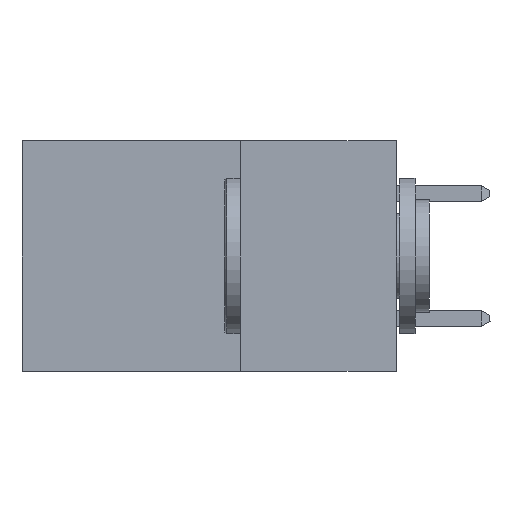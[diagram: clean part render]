
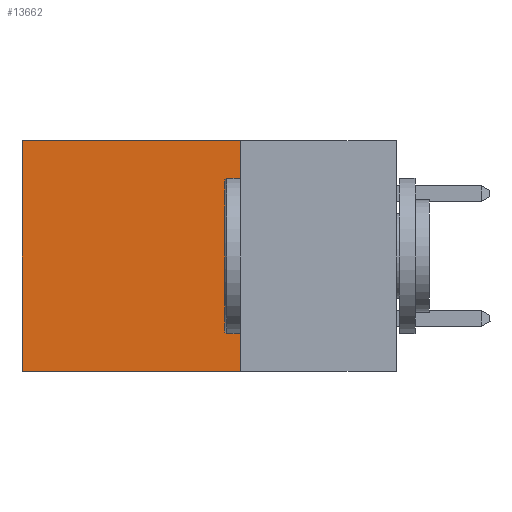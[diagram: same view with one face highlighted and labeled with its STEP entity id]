
A CAD part, left-side view. The second image highlights one B-rep face of the part: STEP entity #13662.
In plain terms, the highlighted planar face has unit normal (-1, 0, 0).
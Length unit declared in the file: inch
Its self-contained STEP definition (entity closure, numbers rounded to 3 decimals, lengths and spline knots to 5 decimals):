
#548 = LINE ( 'NONE', #16639, #19822 ) ;
#828 = PLANE ( 'NONE',  #16685 ) ;
#1911 = CARTESIAN_POINT ( 'NONE',  ( 0.2615, 0.25, -0.37 ) ) ;
#4607 = CARTESIAN_POINT ( 'NONE',  ( 0.2615, 0.25, -0.37 ) ) ;
#5498 = CARTESIAN_POINT ( 'NONE',  ( 0.2615, 0.25, 0. ) ) ;
#6238 = VECTOR ( 'NONE', #6729, 39.37008 ) ;
#6446 = DIRECTION ( 'NONE',  ( 1., 0., 0. ) ) ;
#6654 = CARTESIAN_POINT ( 'NONE',  ( 0.2615, 0.6, -0.37 ) ) ;
#6729 = DIRECTION ( 'NONE',  ( 0., 0., -1. ) ) ;
#7124 = CARTESIAN_POINT ( 'NONE',  ( 0.2615, 0.25, -0.37 ) ) ;
#7173 = VERTEX_POINT ( 'NONE', #5498 ) ;
#7215 = DIRECTION ( 'NONE',  ( 0., 1., 0. ) ) ;
#7771 = LINE ( 'NONE', #1911, #17130 ) ;
#8367 = VECTOR ( 'NONE', #7215, 39.37008 ) ;
#11177 = LINE ( 'NONE', #16035, #6238 ) ;
#12057 = VERTEX_POINT ( 'NONE', #22604 ) ;
#13510 = EDGE_LOOP ( 'NONE', ( #21590, #19247, #22148, #20764 ) ) ;
#13662 = ADVANCED_FACE ( 'NONE', ( #15972 ), #828, .F. ) ;
#13928 = LINE ( 'NONE', #22086, #8367 ) ;
#14014 = EDGE_CURVE ( 'NONE', #7173, #16498, #7771, .T. ) ;
#15007 = VERTEX_POINT ( 'NONE', #6654 ) ;
#15045 = EDGE_CURVE ( 'NONE', #12057, #15007, #11177, .T. ) ;
#15972 = FACE_OUTER_BOUND ( 'NONE', #13510, .T. ) ;
#16035 = CARTESIAN_POINT ( 'NONE',  ( 0.2615, 0.6, -0.37 ) ) ;
#16498 = VERTEX_POINT ( 'NONE', #7124 ) ;
#16639 = CARTESIAN_POINT ( 'NONE',  ( 0.2615, 0.25, 0. ) ) ;
#16685 = AXIS2_PLACEMENT_3D ( 'NONE', #4607, #6446, #19514 ) ;
#16807 = DIRECTION ( 'NONE',  ( 0., 0., -1. ) ) ;
#17130 = VECTOR ( 'NONE', #16807, 39.37008 ) ;
#19247 = ORIENTED_EDGE ( 'NONE', *, *, #21961, .F. ) ;
#19514 = DIRECTION ( 'NONE',  ( 0., 0., -1. ) ) ;
#19822 = VECTOR ( 'NONE', #22207, 39.37008 ) ;
#20764 = ORIENTED_EDGE ( 'NONE', *, *, #20769, .T. ) ;
#20769 = EDGE_CURVE ( 'NONE', #7173, #12057, #548, .T. ) ;
#21590 = ORIENTED_EDGE ( 'NONE', *, *, #15045, .T. ) ;
#21961 = EDGE_CURVE ( 'NONE', #16498, #15007, #13928, .T. ) ;
#22086 = CARTESIAN_POINT ( 'NONE',  ( 0.2615, 0.25, -0.37 ) ) ;
#22148 = ORIENTED_EDGE ( 'NONE', *, *, #14014, .F. ) ;
#22207 = DIRECTION ( 'NONE',  ( 0., 1., 0. ) ) ;
#22604 = CARTESIAN_POINT ( 'NONE',  ( 0.2615, 0.6, 0. ) ) ;
